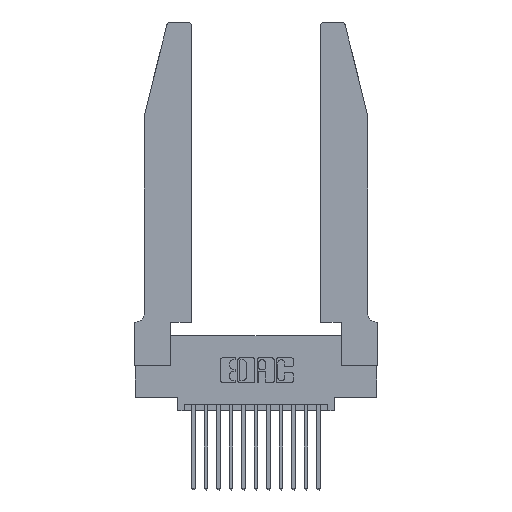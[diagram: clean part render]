
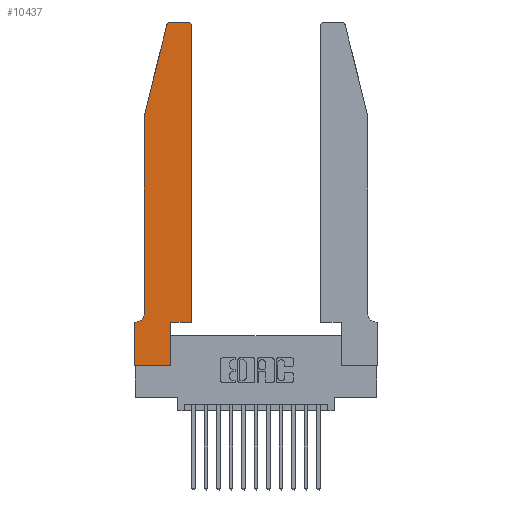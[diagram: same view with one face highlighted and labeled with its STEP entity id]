
A CAD part, top view. The second image highlights one B-rep face of the part: STEP entity #10437.
In plain terms, the highlighted planar face has unit normal (0, 0, 1).
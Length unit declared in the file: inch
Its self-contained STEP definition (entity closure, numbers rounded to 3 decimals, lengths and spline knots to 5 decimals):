
#67 = DIRECTION ( 'NONE',  ( 1., 0., 0. ) ) ;
#77 = ORIENTED_EDGE ( 'NONE', *, *, #15941, .T. ) ;
#155 = CIRCLE ( 'NONE', #11304, 0.03 ) ;
#183 = VERTEX_POINT ( 'NONE', #11495 ) ;
#210 = VERTEX_POINT ( 'NONE', #9824 ) ;
#364 = CARTESIAN_POINT ( 'NONE',  ( 0.2865, 0.35, 0.37 ) ) ;
#516 = ORIENTED_EDGE ( 'NONE', *, *, #10322, .T. ) ;
#637 = VERTEX_POINT ( 'NONE', #15870 ) ;
#747 = CARTESIAN_POINT ( 'NONE',  ( 0.2605, 2.75, 0.37 ) ) ;
#889 = CIRCLE ( 'NONE', #931, 0.07 ) ;
#931 = AXIS2_PLACEMENT_3D ( 'NONE', #13993, #5806, #15366 ) ;
#1000 = CARTESIAN_POINT ( 'NONE',  ( 0.2865, 0., 0.37 ) ) ;
#1008 = EDGE_CURVE ( 'NONE', #17140, #3679, #8743, .T. ) ;
#1105 = EDGE_CURVE ( 'NONE', #183, #16194, #7447, .T. ) ;
#1396 = ORIENTED_EDGE ( 'NONE', *, *, #14478, .T. ) ;
#1891 = EDGE_CURVE ( 'NONE', #3259, #16917, #6791, .T. ) ;
#1997 = CARTESIAN_POINT ( 'NONE',  ( 0.0755, 2., 0.37 ) ) ;
#2228 = DIRECTION ( 'NONE',  ( 1., 0., 0. ) ) ;
#2404 = EDGE_CURVE ( 'NONE', #637, #17140, #6330, .T. ) ;
#2669 = VECTOR ( 'NONE', #3999, 39.37008 ) ;
#2815 = EDGE_CURVE ( 'NONE', #14821, #3259, #17574, .T. ) ;
#2823 = CARTESIAN_POINT ( 'NONE',  ( 0., 0.35, 0.37 ) ) ;
#3259 = VERTEX_POINT ( 'NONE', #1000 ) ;
#3651 = FACE_OUTER_BOUND ( 'NONE', #15649, .T. ) ;
#3679 = VERTEX_POINT ( 'NONE', #9968 ) ;
#3999 = DIRECTION ( 'NONE',  ( 0., 1., 0. ) ) ;
#4606 = CARTESIAN_POINT ( 'NONE',  ( 0., 0., 0.37 ) ) ;
#4666 = ORIENTED_EDGE ( 'NONE', *, *, #1891, .T. ) ;
#4877 = DIRECTION ( 'NONE',  ( 0., 0., 1. ) ) ;
#5502 = VERTEX_POINT ( 'NONE', #11370 ) ;
#5649 = AXIS2_PLACEMENT_3D ( 'NONE', #15100, #4877, #2228 ) ;
#5806 = DIRECTION ( 'NONE',  ( 0., 0., -1. ) ) ;
#6150 = ORIENTED_EDGE ( 'NONE', *, *, #1008, .T. ) ;
#6175 = VECTOR ( 'NONE', #11918, 39.37008 ) ;
#6330 = CIRCLE ( 'NONE', #5649, 0.03 ) ;
#6734 = CARTESIAN_POINT ( 'NONE',  ( 0.4205, 2.72, 0.37 ) ) ;
#6769 = VECTOR ( 'NONE', #14724, 39.37008 ) ;
#6791 = LINE ( 'NONE', #7060, #2669 ) ;
#6993 = EDGE_CURVE ( 'NONE', #7738, #637, #15140, .T. ) ;
#7028 = ORIENTED_EDGE ( 'NONE', *, *, #8433, .T. ) ;
#7060 = CARTESIAN_POINT ( 'NONE',  ( 0.2865, 0.35, 0.37 ) ) ;
#7408 = VECTOR ( 'NONE', #9019, 39.37008 ) ;
#7441 = VECTOR ( 'NONE', #9035, 39.37008 ) ;
#7447 = LINE ( 'NONE', #8330, #14270 ) ;
#7738 = VERTEX_POINT ( 'NONE', #8061 ) ;
#7879 = ORIENTED_EDGE ( 'NONE', *, *, #2815, .T. ) ;
#8061 = CARTESIAN_POINT ( 'NONE',  ( 0.4205, 2.75, 0.37 ) ) ;
#8109 = DIRECTION ( 'NONE',  ( 1., 0., 0. ) ) ;
#8138 = DIRECTION ( 'NONE',  ( 0., -1., 0. ) ) ;
#8234 = EDGE_CURVE ( 'NONE', #3679, #12006, #17584, .T. ) ;
#8324 = ORIENTED_EDGE ( 'NONE', *, *, #17713, .T. ) ;
#8330 = CARTESIAN_POINT ( 'NONE',  ( 0.4505, 0.35, 0.37 ) ) ;
#8379 = DIRECTION ( 'NONE',  ( 0., 0., 1. ) ) ;
#8433 = EDGE_CURVE ( 'NONE', #12006, #5502, #889, .T. ) ;
#8743 = LINE ( 'NONE', #1997, #9169 ) ;
#8944 = ORIENTED_EDGE ( 'NONE', *, *, #2404, .T. ) ;
#9019 = DIRECTION ( 'NONE',  ( 1., 0., 0. ) ) ;
#9035 = DIRECTION ( 'NONE',  ( -1., 0., 0. ) ) ;
#9169 = VECTOR ( 'NONE', #15867, 39.37008 ) ;
#9229 = CARTESIAN_POINT ( 'NONE',  ( 0., 0., 0.37 ) ) ;
#9481 = LINE ( 'NONE', #16294, #13112 ) ;
#9693 = DIRECTION ( 'NONE',  ( 1., 0., 0. ) ) ;
#9824 = CARTESIAN_POINT ( 'NONE',  ( 0., 0.35, 0.37 ) ) ;
#9968 = CARTESIAN_POINT ( 'NONE',  ( 0.0755, 2., 0.37 ) ) ;
#10243 = ORIENTED_EDGE ( 'NONE', *, *, #8234, .T. ) ;
#10322 = EDGE_CURVE ( 'NONE', #210, #14821, #9481, .T. ) ;
#10336 = CARTESIAN_POINT ( 'NONE',  ( 0.4505, 0.35, 0.37 ) ) ;
#10437 = ADVANCED_FACE ( 'NONE', ( #3651 ), #16514, .T. ) ;
#10543 = CARTESIAN_POINT ( 'NONE',  ( 0.0755, 0.35, 0.37 ) ) ;
#10678 = CARTESIAN_POINT ( 'NONE',  ( 0.0755, 2., 0.37 ) ) ;
#10689 = DIRECTION ( 'NONE',  ( 0., 1., 0. ) ) ;
#11030 = CARTESIAN_POINT ( 'NONE',  ( 0.4505, 2.72, 0.37 ) ) ;
#11068 = LINE ( 'NONE', #10336, #7408 ) ;
#11304 = AXIS2_PLACEMENT_3D ( 'NONE', #6734, #16255, #8109 ) ;
#11370 = CARTESIAN_POINT ( 'NONE',  ( 0.0055, 0.35, 0.37 ) ) ;
#11495 = CARTESIAN_POINT ( 'NONE',  ( 0.4505, 0.35, 0.37 ) ) ;
#11824 = CARTESIAN_POINT ( 'NONE',  ( 0.25487, 2.72718, 0.37 ) ) ;
#11918 = DIRECTION ( 'NONE',  ( -1., 0., 0. ) ) ;
#11960 = ORIENTED_EDGE ( 'NONE', *, *, #1105, .T. ) ;
#12006 = VERTEX_POINT ( 'NONE', #14331 ) ;
#13112 = VECTOR ( 'NONE', #8138, 39.37008 ) ;
#13461 = LINE ( 'NONE', #10543, #6175 ) ;
#13993 = CARTESIAN_POINT ( 'NONE',  ( 0.0055, 0.42, 0.37 ) ) ;
#14270 = VECTOR ( 'NONE', #10689, 39.37008 ) ;
#14331 = CARTESIAN_POINT ( 'NONE',  ( 0.0755, 0.42, 0.37 ) ) ;
#14478 = EDGE_CURVE ( 'NONE', #16194, #7738, #155, .T. ) ;
#14724 = DIRECTION ( 'NONE',  ( 0., -1., 0. ) ) ;
#14821 = VERTEX_POINT ( 'NONE', #9229 ) ;
#14877 = VECTOR ( 'NONE', #9693, 39.37008 ) ;
#15100 = CARTESIAN_POINT ( 'NONE',  ( 0.284, 2.72, 0.37 ) ) ;
#15140 = LINE ( 'NONE', #747, #7441 ) ;
#15366 = DIRECTION ( 'NONE',  ( -1., 0., 0. ) ) ;
#15649 = EDGE_LOOP ( 'NONE', ( #15768, #8944, #6150, #10243, #7028, #77, #516, #7879, #4666, #8324, #11960, #1396 ) ) ;
#15768 = ORIENTED_EDGE ( 'NONE', *, *, #6993, .T. ) ;
#15784 = AXIS2_PLACEMENT_3D ( 'NONE', #2823, #8379, #67 ) ;
#15867 = DIRECTION ( 'NONE',  ( -0.239, -0.971, 0. ) ) ;
#15870 = CARTESIAN_POINT ( 'NONE',  ( 0.284, 2.75, 0.37 ) ) ;
#15941 = EDGE_CURVE ( 'NONE', #5502, #210, #13461, .T. ) ;
#16194 = VERTEX_POINT ( 'NONE', #11030 ) ;
#16255 = DIRECTION ( 'NONE',  ( 0., 0., 1. ) ) ;
#16294 = CARTESIAN_POINT ( 'NONE',  ( 0., 0., 0.37 ) ) ;
#16514 = PLANE ( 'NONE',  #15784 ) ;
#16917 = VERTEX_POINT ( 'NONE', #364 ) ;
#17140 = VERTEX_POINT ( 'NONE', #11824 ) ;
#17574 = LINE ( 'NONE', #4606, #14877 ) ;
#17584 = LINE ( 'NONE', #10678, #6769 ) ;
#17713 = EDGE_CURVE ( 'NONE', #16917, #183, #11068, .T. ) ;
